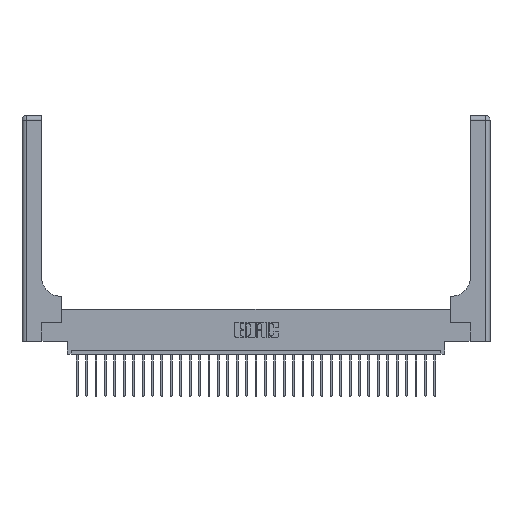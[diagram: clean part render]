
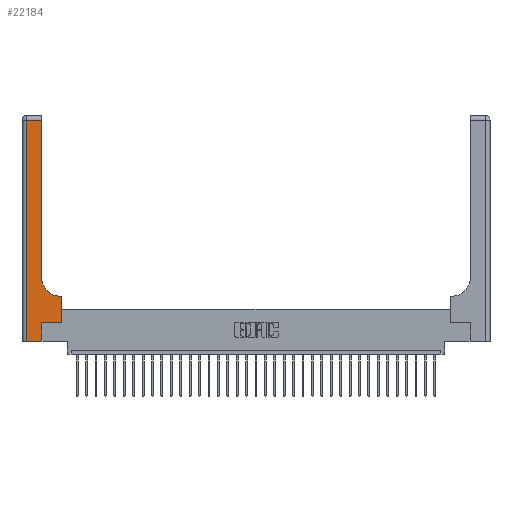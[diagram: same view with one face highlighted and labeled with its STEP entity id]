
A CAD part, top view. The second image highlights one B-rep face of the part: STEP entity #22184.
In plain terms, the highlighted planar face has unit normal (0, 0, 1).
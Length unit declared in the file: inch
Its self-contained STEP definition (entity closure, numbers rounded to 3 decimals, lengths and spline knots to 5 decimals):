
#778 = LINE ( 'NONE', #2942, #18387 ) ;
#1591 = DIRECTION ( 'NONE',  ( -1., 0., 0. ) ) ;
#2571 = DIRECTION ( 'NONE',  ( 0., 0., -1. ) ) ;
#2877 = VECTOR ( 'NONE', #6091, 39.37008 ) ;
#2942 = CARTESIAN_POINT ( 'NONE',  ( 0.265, 0.25, 0.37 ) ) ;
#3337 = VERTEX_POINT ( 'NONE', #4129 ) ;
#4129 = CARTESIAN_POINT ( 'NONE',  ( 0.06, 2.94, 0.37 ) ) ;
#4331 = ORIENTED_EDGE ( 'NONE', *, *, #11569, .T. ) ;
#4362 = CARTESIAN_POINT ( 'NONE',  ( 0., 2.94, 0.37 ) ) ;
#4568 = VERTEX_POINT ( 'NONE', #24580 ) ;
#4992 = CARTESIAN_POINT ( 'NONE',  ( 0.528, 0.25, 0.37 ) ) ;
#5002 = LINE ( 'NONE', #20099, #14832 ) ;
#5658 = DIRECTION ( 'NONE',  ( 0., 0., -1. ) ) ;
#6091 = DIRECTION ( 'NONE',  ( 0., 1., 0. ) ) ;
#7138 = LINE ( 'NONE', #4992, #9107 ) ;
#7355 = PLANE ( 'NONE',  #17688 ) ;
#8220 = CARTESIAN_POINT ( 'NONE',  ( 0.26, 3., 0.37 ) ) ;
#8282 = VERTEX_POINT ( 'NONE', #19019 ) ;
#8781 = VECTOR ( 'NONE', #15911, 39.37008 ) ;
#9107 = VECTOR ( 'NONE', #12211, 39.37008 ) ;
#9147 = VERTEX_POINT ( 'NONE', #28235 ) ;
#9237 = EDGE_CURVE ( 'NONE', #8282, #19113, #14447, .T. ) ;
#9613 = LINE ( 'NONE', #18570, #28462 ) ;
#10036 = EDGE_CURVE ( 'NONE', #22813, #4568, #7138, .T. ) ;
#10265 = CARTESIAN_POINT ( 'NONE',  ( 0.51, 0.85, 0.37 ) ) ;
#10482 = LINE ( 'NONE', #24932, #22158 ) ;
#10989 = CARTESIAN_POINT ( 'NONE',  ( 0.528, 0.25, 0.37 ) ) ;
#11507 = DIRECTION ( 'NONE',  ( -1., 0., 0. ) ) ;
#11563 = LINE ( 'NONE', #4362, #8781 ) ;
#11569 = EDGE_CURVE ( 'NONE', #26684, #3337, #11563, .T. ) ;
#11908 = EDGE_CURVE ( 'NONE', #3337, #26925, #10482, .T. ) ;
#12066 = VECTOR ( 'NONE', #20944, 39.37008 ) ;
#12211 = DIRECTION ( 'NONE',  ( 0., 1., 0. ) ) ;
#12717 = EDGE_CURVE ( 'NONE', #4568, #8282, #5002, .T. ) ;
#12726 = DIRECTION ( 'NONE',  ( 1., 0., 0. ) ) ;
#13348 = ORIENTED_EDGE ( 'NONE', *, *, #9237, .T. ) ;
#13493 = EDGE_LOOP ( 'NONE', ( #21043, #4331, #19296, #19449, #28612, #18008, #29345, #29295, #13348 ) ) ;
#14133 = CARTESIAN_POINT ( 'NONE',  ( 0.06, 0., 0.37 ) ) ;
#14262 = FACE_OUTER_BOUND ( 'NONE', #13493, .T. ) ;
#14447 = CIRCLE ( 'NONE', #28190, 0.25 ) ;
#14832 = VECTOR ( 'NONE', #1591, 39.37008 ) ;
#14878 = LINE ( 'NONE', #8220, #2877 ) ;
#15911 = DIRECTION ( 'NONE',  ( -1., 0., 0. ) ) ;
#16427 = DIRECTION ( 'NONE',  ( 0., 1., 0. ) ) ;
#16464 = CARTESIAN_POINT ( 'NONE',  ( 0., 3., 0.37 ) ) ;
#17075 = EDGE_CURVE ( 'NONE', #26925, #23061, #26918, .T. ) ;
#17413 = DIRECTION ( 'NONE',  ( 0., -1., 0. ) ) ;
#17688 = AXIS2_PLACEMENT_3D ( 'NONE', #16464, #2571, #11507 ) ;
#18008 = ORIENTED_EDGE ( 'NONE', *, *, #24770, .T. ) ;
#18387 = VECTOR ( 'NONE', #29054, 39.37008 ) ;
#18570 = CARTESIAN_POINT ( 'NONE',  ( 0.265, 0., 0.37 ) ) ;
#19019 = CARTESIAN_POINT ( 'NONE',  ( 0.51, 0.6, 0.37 ) ) ;
#19113 = VERTEX_POINT ( 'NONE', #22999 ) ;
#19296 = ORIENTED_EDGE ( 'NONE', *, *, #11908, .T. ) ;
#19449 = ORIENTED_EDGE ( 'NONE', *, *, #17075, .T. ) ;
#20099 = CARTESIAN_POINT ( 'NONE',  ( 0.26, 0.6, 0.37 ) ) ;
#20944 = DIRECTION ( 'NONE',  ( 1., 0., 0. ) ) ;
#21043 = ORIENTED_EDGE ( 'NONE', *, *, #26262, .T. ) ;
#22158 = VECTOR ( 'NONE', #17413, 39.37008 ) ;
#22184 = ADVANCED_FACE ( 'NONE', ( #14262 ), #7355, .F. ) ;
#22602 = EDGE_CURVE ( 'NONE', #23061, #9147, #9613, .T. ) ;
#22813 = VERTEX_POINT ( 'NONE', #10989 ) ;
#22999 = CARTESIAN_POINT ( 'NONE',  ( 0.26, 0.85, 0.37 ) ) ;
#23061 = VERTEX_POINT ( 'NONE', #29084 ) ;
#24580 = CARTESIAN_POINT ( 'NONE',  ( 0.528, 0.6, 0.37 ) ) ;
#24619 = CARTESIAN_POINT ( 'NONE',  ( 0., 0., 0.37 ) ) ;
#24770 = EDGE_CURVE ( 'NONE', #9147, #22813, #778, .T. ) ;
#24932 = CARTESIAN_POINT ( 'NONE',  ( 0.06, 3., 0.37 ) ) ;
#26262 = EDGE_CURVE ( 'NONE', #19113, #26684, #14878, .T. ) ;
#26684 = VERTEX_POINT ( 'NONE', #28642 ) ;
#26918 = LINE ( 'NONE', #24619, #12066 ) ;
#26925 = VERTEX_POINT ( 'NONE', #14133 ) ;
#28190 = AXIS2_PLACEMENT_3D ( 'NONE', #10265, #5658, #12726 ) ;
#28235 = CARTESIAN_POINT ( 'NONE',  ( 0.265, 0.25, 0.37 ) ) ;
#28462 = VECTOR ( 'NONE', #16427, 39.37008 ) ;
#28612 = ORIENTED_EDGE ( 'NONE', *, *, #22602, .T. ) ;
#28642 = CARTESIAN_POINT ( 'NONE',  ( 0.26, 2.94, 0.37 ) ) ;
#29054 = DIRECTION ( 'NONE',  ( 1., 0., 0. ) ) ;
#29084 = CARTESIAN_POINT ( 'NONE',  ( 0.265, 0., 0.37 ) ) ;
#29295 = ORIENTED_EDGE ( 'NONE', *, *, #12717, .T. ) ;
#29345 = ORIENTED_EDGE ( 'NONE', *, *, #10036, .T. ) ;
